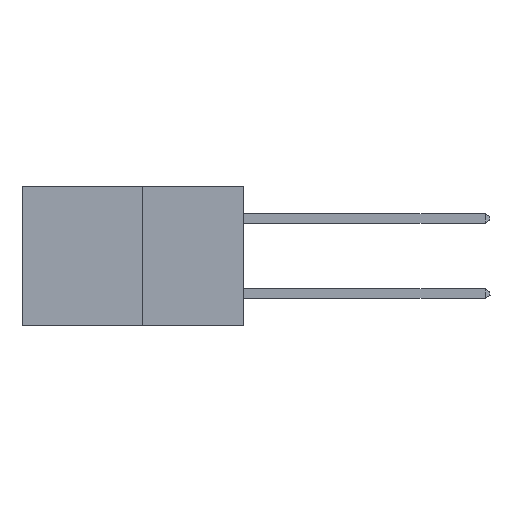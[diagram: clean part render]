
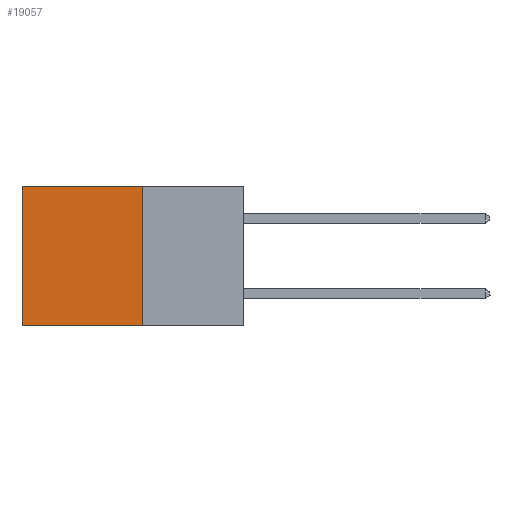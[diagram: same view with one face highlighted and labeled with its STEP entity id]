
A CAD part, left-side view. The second image highlights one B-rep face of the part: STEP entity #19057.
In plain terms, the highlighted planar face has unit normal (-1, 0, 0).
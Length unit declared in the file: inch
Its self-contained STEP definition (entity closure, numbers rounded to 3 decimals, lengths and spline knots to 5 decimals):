
#240 = LINE ( 'NONE', #26555, #5365 ) ;
#445 = VECTOR ( 'NONE', #22430, 39.37008 ) ;
#1807 = VECTOR ( 'NONE', #6382, 39.37008 ) ;
#2186 = ORIENTED_EDGE ( 'NONE', *, *, #23647, .F. ) ;
#2396 = CARTESIAN_POINT ( 'NONE',  ( 0.277, 0.27, 0. ) ) ;
#4056 = VECTOR ( 'NONE', #9237, 39.37008 ) ;
#4199 = CARTESIAN_POINT ( 'NONE',  ( 0.277, 0.27, -0.37 ) ) ;
#4739 = LINE ( 'NONE', #4843, #4056 ) ;
#4843 = CARTESIAN_POINT ( 'NONE',  ( 0.277, 0.27, 0. ) ) ;
#5365 = VECTOR ( 'NONE', #7453, 39.37008 ) ;
#6382 = DIRECTION ( 'NONE',  ( 0., 1., 0. ) ) ;
#6995 = PLANE ( 'NONE',  #22821 ) ;
#7453 = DIRECTION ( 'NONE',  ( 0., 0., -1. ) ) ;
#7580 = LINE ( 'NONE', #4199, #1807 ) ;
#8388 = FACE_OUTER_BOUND ( 'NONE', #18479, .T. ) ;
#9221 = DIRECTION ( 'NONE',  ( 1., 0., 0. ) ) ;
#9237 = DIRECTION ( 'NONE',  ( 0., 1., 0. ) ) ;
#9703 = VERTEX_POINT ( 'NONE', #13986 ) ;
#10629 = EDGE_CURVE ( 'NONE', #15436, #10708, #4739, .T. ) ;
#10708 = VERTEX_POINT ( 'NONE', #11497 ) ;
#11497 = CARTESIAN_POINT ( 'NONE',  ( 0.277, 0.59, 0. ) ) ;
#11509 = EDGE_CURVE ( 'NONE', #10708, #13013, #240, .T. ) ;
#11661 = ORIENTED_EDGE ( 'NONE', *, *, #10629, .T. ) ;
#12509 = CARTESIAN_POINT ( 'NONE',  ( 0.277, 0.59, -0.37 ) ) ;
#12536 = ORIENTED_EDGE ( 'NONE', *, *, #11509, .T. ) ;
#13013 = VERTEX_POINT ( 'NONE', #12509 ) ;
#13986 = CARTESIAN_POINT ( 'NONE',  ( 0.277, 0.27, -0.37 ) ) ;
#14369 = ORIENTED_EDGE ( 'NONE', *, *, #20455, .F. ) ;
#15436 = VERTEX_POINT ( 'NONE', #2396 ) ;
#18479 = EDGE_LOOP ( 'NONE', ( #12536, #2186, #14369, #11661 ) ) ;
#19057 = ADVANCED_FACE ( 'NONE', ( #8388 ), #6995, .F. ) ;
#19771 = CARTESIAN_POINT ( 'NONE',  ( 0.277, 0.27, -0.37 ) ) ;
#20455 = EDGE_CURVE ( 'NONE', #15436, #9703, #23925, .T. ) ;
#22430 = DIRECTION ( 'NONE',  ( 0., 0., -1. ) ) ;
#22821 = AXIS2_PLACEMENT_3D ( 'NONE', #19771, #9221, #24032 ) ;
#23647 = EDGE_CURVE ( 'NONE', #9703, #13013, #7580, .T. ) ;
#23925 = LINE ( 'NONE', #24657, #445 ) ;
#24032 = DIRECTION ( 'NONE',  ( 0., 0., -1. ) ) ;
#24657 = CARTESIAN_POINT ( 'NONE',  ( 0.277, 0.27, -0.37 ) ) ;
#26555 = CARTESIAN_POINT ( 'NONE',  ( 0.277, 0.59, -0.37 ) ) ;
